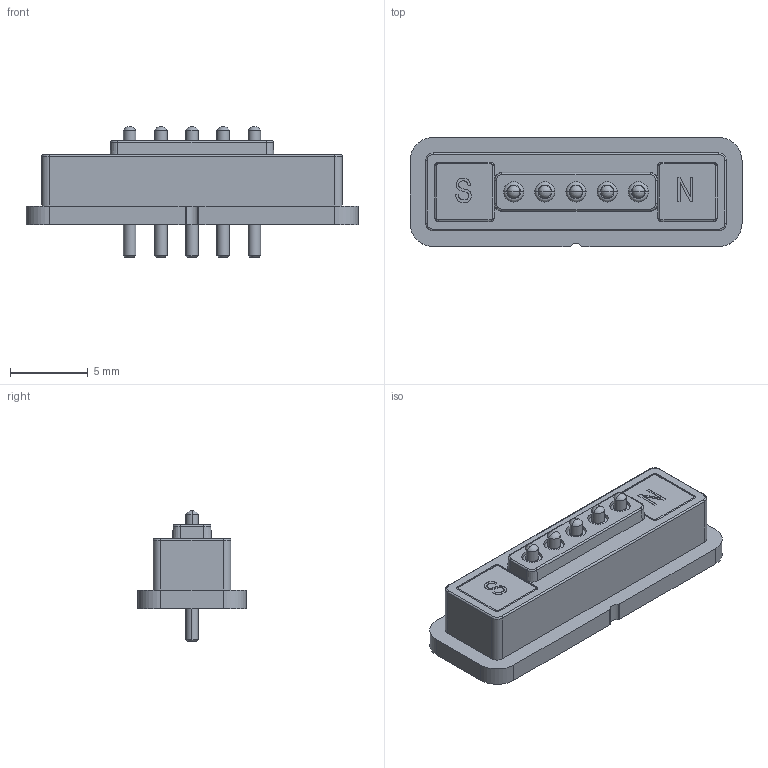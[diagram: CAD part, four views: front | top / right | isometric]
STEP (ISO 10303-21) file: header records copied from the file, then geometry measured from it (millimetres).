
FILE_DESCRIPTION (( 'STEP AP214' ), '1' );
FILE_NAME ('685J0521251110E.STEP', '2023-04-13T19:24:53', ( '' ), ( '' ), 'SwSTEP 2.0', 'SolidWorks 2020', '' );
FILE_SCHEMA (( 'AUTOMOTIVE_DESIGN' ));
Length unit declared in the file: millimetre
Products named in the file (1): 685J0521251110E
Bounding box: 21.3 x 7 x 8.4 mm (x, y, z)
Volume: 473 mm3; surface area: 814.4 mm2
Topology: 6 solids, 13 shells, 304 faces, 674 edges, 414 vertices
Faces by surface type: cylinder 121, plane 96, cone 29, bspline 26, torus 22, sphere 10
Entity records: 11558 total; most frequent: CARTESIAN_POINT 2409, DIRECTION 1520, ORIENTED_EDGE 1348, EDGE_CURVE 674, AXIS2_PLACEMENT_3D 597, VERTEX_POINT 414, EDGE_LOOP 336, VECTOR 326
